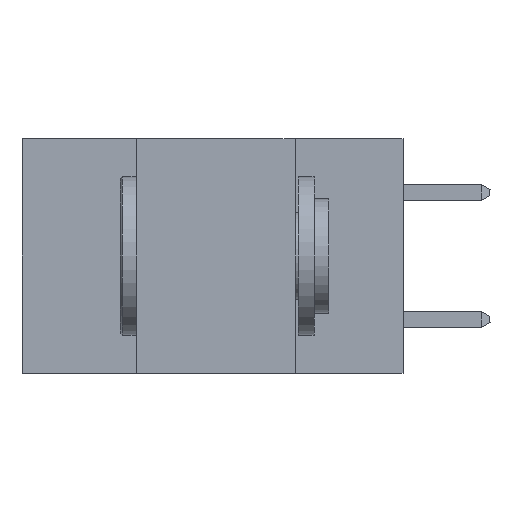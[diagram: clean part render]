
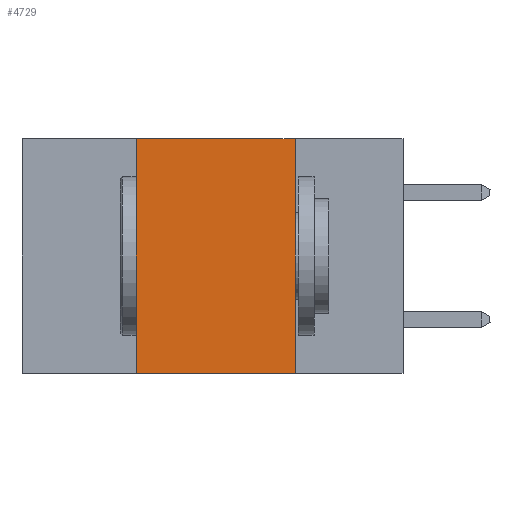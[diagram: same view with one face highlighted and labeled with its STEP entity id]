
A CAD part, left-side view. The second image highlights one B-rep face of the part: STEP entity #4729.
In plain terms, the highlighted planar face has unit normal (-1, 0, 0).
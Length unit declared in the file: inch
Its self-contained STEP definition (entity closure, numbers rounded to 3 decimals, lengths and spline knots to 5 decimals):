
#513 = CARTESIAN_POINT ( 'NONE',  ( 0., 0.17, 0. ) ) ;
#1274 = LINE ( 'NONE', #20379, #15284 ) ;
#1319 = DIRECTION ( 'NONE',  ( 0., 0., -1. ) ) ;
#2525 = EDGE_LOOP ( 'NONE', ( #8336, #20672, #11779, #19061 ) ) ;
#3001 = VERTEX_POINT ( 'NONE', #10221 ) ;
#3087 = DIRECTION ( 'NONE',  ( 0., 0., -1. ) ) ;
#3107 = DIRECTION ( 'NONE',  ( 1., 0., 0. ) ) ;
#3139 = CARTESIAN_POINT ( 'NONE',  ( 0., 0.6, 0. ) ) ;
#3166 = PLANE ( 'NONE',  #20540 ) ;
#4729 = ADVANCED_FACE ( 'NONE', ( #10561 ), #3166, .F. ) ;
#4821 = EDGE_CURVE ( 'NONE', #3001, #11991, #9983, .T. ) ;
#5465 = CARTESIAN_POINT ( 'NONE',  ( 0., 0.42, -0.37 ) ) ;
#5630 = EDGE_CURVE ( 'NONE', #11783, #3001, #1274, .T. ) ;
#6304 = CARTESIAN_POINT ( 'NONE',  ( 0., 0.42, 0. ) ) ;
#6742 = DIRECTION ( 'NONE',  ( 0., -1., 0. ) ) ;
#7527 = DIRECTION ( 'NONE',  ( 0., 0., 1. ) ) ;
#7844 = DIRECTION ( 'NONE',  ( 0., -1., 0. ) ) ;
#8336 = ORIENTED_EDGE ( 'NONE', *, *, #4821, .F. ) ;
#8696 = CARTESIAN_POINT ( 'NONE',  ( 0., 0.17, -0.37 ) ) ;
#9759 = LINE ( 'NONE', #13961, #11765 ) ;
#9983 = LINE ( 'NONE', #513, #17880 ) ;
#10221 = CARTESIAN_POINT ( 'NONE',  ( 0., 0.17, 0. ) ) ;
#10400 = VECTOR ( 'NONE', #7527, 39.37008 ) ;
#10561 = FACE_OUTER_BOUND ( 'NONE', #2525, .T. ) ;
#11765 = VECTOR ( 'NONE', #6742, 39.37008 ) ;
#11779 = ORIENTED_EDGE ( 'NONE', *, *, #12205, .F. ) ;
#11783 = VERTEX_POINT ( 'NONE', #6304 ) ;
#11991 = VERTEX_POINT ( 'NONE', #8696 ) ;
#12205 = EDGE_CURVE ( 'NONE', #18276, #11783, #15165, .T. ) ;
#13961 = CARTESIAN_POINT ( 'NONE',  ( 0., 0.6, -0.37 ) ) ;
#15165 = LINE ( 'NONE', #19993, #10400 ) ;
#15284 = VECTOR ( 'NONE', #7844, 39.37008 ) ;
#16854 = EDGE_CURVE ( 'NONE', #18276, #11991, #9759, .T. ) ;
#17880 = VECTOR ( 'NONE', #1319, 39.37008 ) ;
#18276 = VERTEX_POINT ( 'NONE', #5465 ) ;
#19061 = ORIENTED_EDGE ( 'NONE', *, *, #16854, .T. ) ;
#19993 = CARTESIAN_POINT ( 'NONE',  ( 0., 0.42, 0. ) ) ;
#20379 = CARTESIAN_POINT ( 'NONE',  ( 0., 0.6, 0. ) ) ;
#20540 = AXIS2_PLACEMENT_3D ( 'NONE', #3139, #3107, #3087 ) ;
#20672 = ORIENTED_EDGE ( 'NONE', *, *, #5630, .F. ) ;
